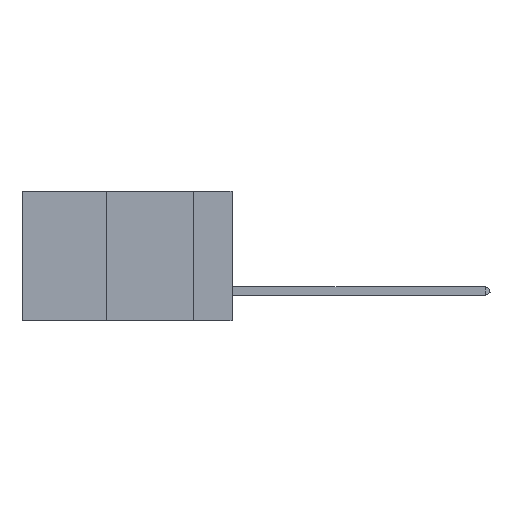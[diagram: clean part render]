
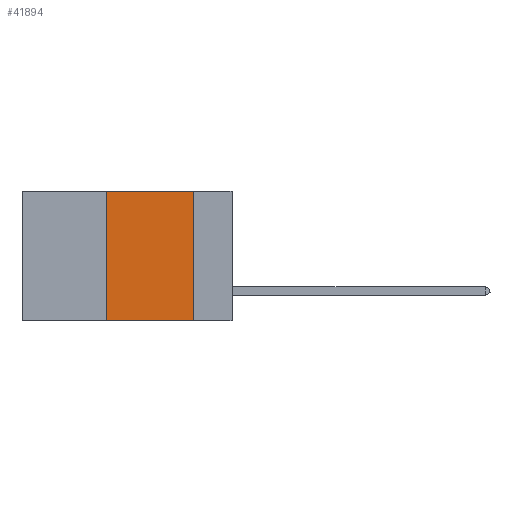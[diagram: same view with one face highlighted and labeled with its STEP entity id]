
A CAD part, left-side view. The second image highlights one B-rep face of the part: STEP entity #41894.
In plain terms, the highlighted planar face has unit normal (-1, 0, 0).
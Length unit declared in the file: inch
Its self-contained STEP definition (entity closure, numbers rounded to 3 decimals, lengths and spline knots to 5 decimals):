
#1034 = AXIS2_PLACEMENT_3D ( 'NONE', #33331, #36792, #25939 ) ;
#1611 = DIRECTION ( 'NONE',  ( 0., 0., -1. ) ) ;
#2162 = VECTOR ( 'NONE', #34097, 39.37008 ) ;
#2194 = ORIENTED_EDGE ( 'NONE', *, *, #22583, .T. ) ;
#2710 = CARTESIAN_POINT ( 'NONE',  ( 0., 0.6, -0.37 ) ) ;
#2865 = DIRECTION ( 'NONE',  ( 0., 0., 1. ) ) ;
#4949 = CARTESIAN_POINT ( 'NONE',  ( 0., 0.36, -0.37 ) ) ;
#5174 = CARTESIAN_POINT ( 'NONE',  ( 0., 0.11, 0. ) ) ;
#5294 = LINE ( 'NONE', #2710, #2162 ) ;
#5611 = ORIENTED_EDGE ( 'NONE', *, *, #34137, .F. ) ;
#9161 = EDGE_CURVE ( 'NONE', #23538, #28522, #30557, .T. ) ;
#9429 = EDGE_LOOP ( 'NONE', ( #27981, #5611, #45017, #2194 ) ) ;
#12335 = PLANE ( 'NONE',  #1034 ) ;
#12573 = VERTEX_POINT ( 'NONE', #5174 ) ;
#13032 = CARTESIAN_POINT ( 'NONE',  ( 0., 0.36, 0. ) ) ;
#14630 = VECTOR ( 'NONE', #1611, 39.37008 ) ;
#15331 = FACE_OUTER_BOUND ( 'NONE', #9429, .T. ) ;
#16254 = VECTOR ( 'NONE', #2865, 39.37008 ) ;
#22129 = CARTESIAN_POINT ( 'NONE',  ( 0., 0.11, 0. ) ) ;
#22226 = EDGE_CURVE ( 'NONE', #12573, #28961, #29271, .T. ) ;
#22583 = EDGE_CURVE ( 'NONE', #23538, #28961, #5294, .T. ) ;
#23538 = VERTEX_POINT ( 'NONE', #4949 ) ;
#25180 = CARTESIAN_POINT ( 'NONE',  ( 0., 0.36, 0. ) ) ;
#25939 = DIRECTION ( 'NONE',  ( 0., 0., -1. ) ) ;
#26484 = VECTOR ( 'NONE', #42214, 39.37008 ) ;
#27981 = ORIENTED_EDGE ( 'NONE', *, *, #22226, .F. ) ;
#28522 = VERTEX_POINT ( 'NONE', #25180 ) ;
#28961 = VERTEX_POINT ( 'NONE', #32223 ) ;
#29271 = LINE ( 'NONE', #22129, #14630 ) ;
#30557 = LINE ( 'NONE', #13032, #16254 ) ;
#30916 = CARTESIAN_POINT ( 'NONE',  ( 0., 0.6, 0. ) ) ;
#32223 = CARTESIAN_POINT ( 'NONE',  ( 0., 0.11, -0.37 ) ) ;
#33331 = CARTESIAN_POINT ( 'NONE',  ( 0., 0.6, 0. ) ) ;
#34097 = DIRECTION ( 'NONE',  ( 0., -1., 0. ) ) ;
#34137 = EDGE_CURVE ( 'NONE', #28522, #12573, #38748, .T. ) ;
#36792 = DIRECTION ( 'NONE',  ( 1., 0., 0. ) ) ;
#38748 = LINE ( 'NONE', #30916, #26484 ) ;
#41894 = ADVANCED_FACE ( 'NONE', ( #15331 ), #12335, .F. ) ;
#42214 = DIRECTION ( 'NONE',  ( 0., -1., 0. ) ) ;
#45017 = ORIENTED_EDGE ( 'NONE', *, *, #9161, .F. ) ;
